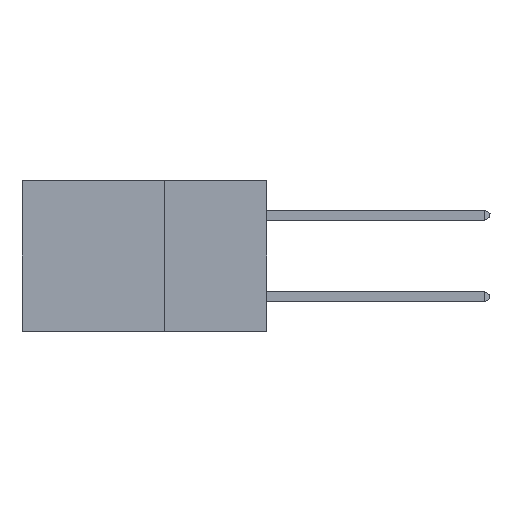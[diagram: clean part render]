
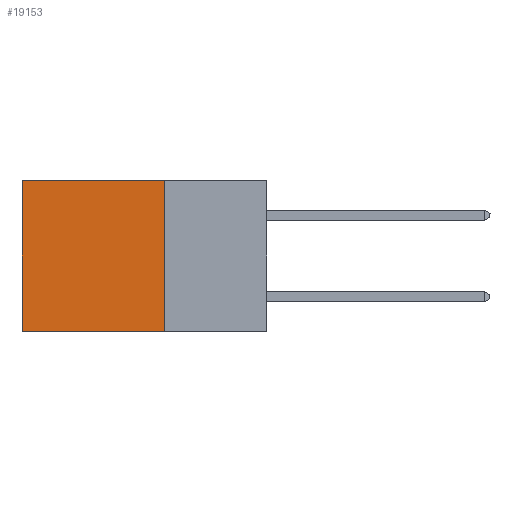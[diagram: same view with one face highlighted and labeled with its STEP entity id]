
A CAD part, left-side view. The second image highlights one B-rep face of the part: STEP entity #19153.
In plain terms, the highlighted planar face has unit normal (-1, 0, 0).
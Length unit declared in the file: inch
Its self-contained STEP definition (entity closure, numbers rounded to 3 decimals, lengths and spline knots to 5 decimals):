
#432 = DIRECTION ( 'NONE',  ( 0., 0., -1. ) ) ;
#1022 = LINE ( 'NONE', #12548, #22616 ) ;
#1771 = DIRECTION ( 'NONE',  ( 0., 0., -1. ) ) ;
#1878 = VECTOR ( 'NONE', #19300, 39.37008 ) ;
#4910 = CARTESIAN_POINT ( 'NONE',  ( 0.2875, 0.6, -0.37 ) ) ;
#5044 = CARTESIAN_POINT ( 'NONE',  ( 0.2875, 0.6, 0. ) ) ;
#5747 = PLANE ( 'NONE',  #31374 ) ;
#7671 = CARTESIAN_POINT ( 'NONE',  ( 0.2875, 0.25, -0.37 ) ) ;
#8191 = EDGE_CURVE ( 'NONE', #30086, #10831, #1022, .T. ) ;
#9143 = DIRECTION ( 'NONE',  ( 1., 0., 0. ) ) ;
#10831 = VERTEX_POINT ( 'NONE', #34601 ) ;
#10859 = DIRECTION ( 'NONE',  ( 0., 1., 0. ) ) ;
#12548 = CARTESIAN_POINT ( 'NONE',  ( 0.2875, 0.25, 0. ) ) ;
#12664 = VECTOR ( 'NONE', #34474, 39.37008 ) ;
#12917 = VERTEX_POINT ( 'NONE', #31153 ) ;
#12976 = VERTEX_POINT ( 'NONE', #4910 ) ;
#13793 = EDGE_LOOP ( 'NONE', ( #18265, #23352, #27660, #28451 ) ) ;
#16824 = LINE ( 'NONE', #36815, #1878 ) ;
#18265 = ORIENTED_EDGE ( 'NONE', *, *, #24083, .T. ) ;
#19153 = ADVANCED_FACE ( 'NONE', ( #31617 ), #5747, .F. ) ;
#19300 = DIRECTION ( 'NONE',  ( 0., 1., 0. ) ) ;
#19383 = LINE ( 'NONE', #7671, #32975 ) ;
#22616 = VECTOR ( 'NONE', #1771, 39.37008 ) ;
#23150 = CARTESIAN_POINT ( 'NONE',  ( 0.2875, 0.25, 0. ) ) ;
#23352 = ORIENTED_EDGE ( 'NONE', *, *, #34033, .F. ) ;
#24083 = EDGE_CURVE ( 'NONE', #12917, #12976, #34121, .T. ) ;
#25486 = EDGE_CURVE ( 'NONE', #30086, #12917, #16824, .T. ) ;
#27660 = ORIENTED_EDGE ( 'NONE', *, *, #8191, .F. ) ;
#28451 = ORIENTED_EDGE ( 'NONE', *, *, #25486, .T. ) ;
#28787 = CARTESIAN_POINT ( 'NONE',  ( 0.2875, 0.25, 0. ) ) ;
#30086 = VERTEX_POINT ( 'NONE', #23150 ) ;
#31153 = CARTESIAN_POINT ( 'NONE',  ( 0.2875, 0.6, 0. ) ) ;
#31374 = AXIS2_PLACEMENT_3D ( 'NONE', #28787, #9143, #432 ) ;
#31617 = FACE_OUTER_BOUND ( 'NONE', #13793, .T. ) ;
#32975 = VECTOR ( 'NONE', #10859, 39.37008 ) ;
#34033 = EDGE_CURVE ( 'NONE', #10831, #12976, #19383, .T. ) ;
#34121 = LINE ( 'NONE', #5044, #12664 ) ;
#34474 = DIRECTION ( 'NONE',  ( 0., 0., -1. ) ) ;
#34601 = CARTESIAN_POINT ( 'NONE',  ( 0.2875, 0.25, -0.37 ) ) ;
#36815 = CARTESIAN_POINT ( 'NONE',  ( 0.2875, 0.25, 0. ) ) ;
